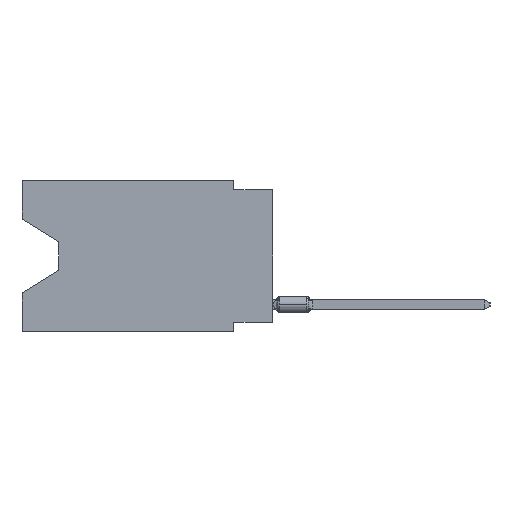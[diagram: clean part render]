
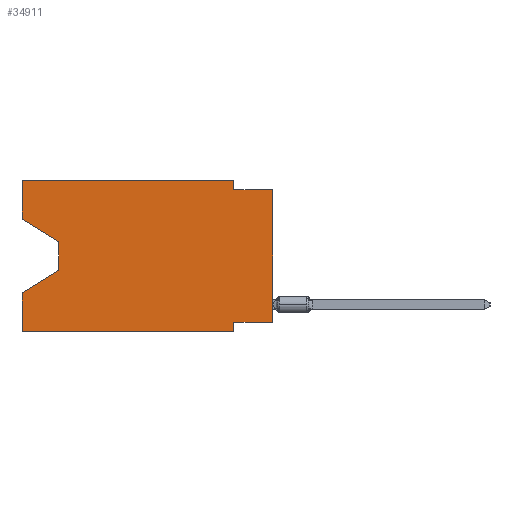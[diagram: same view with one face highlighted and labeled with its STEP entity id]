
A CAD part, left-side view. The second image highlights one B-rep face of the part: STEP entity #34911.
In plain terms, the highlighted planar face has unit normal (-1, 0, 0).
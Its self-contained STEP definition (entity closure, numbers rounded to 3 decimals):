
#473 = LINE ( 'NONE', #30649, #62997 ) ;
#828 = LINE ( 'NONE', #5421, #24261 ) ;
#2259 = CARTESIAN_POINT ( 'NONE',  ( 0., 16.383, -9.906 ) ) ;
#2526 = EDGE_CURVE ( 'NONE', #58920, #43027, #473, .T. ) ;
#2875 = EDGE_LOOP ( 'NONE', ( #43694, #42628, #30547, #45548, #38217, #61983, #20829, #27153, #55555, #23919, #49147, #15992 ) ) ;
#4630 = AXIS2_PLACEMENT_3D ( 'NONE', #52921, #58157, #6998 ) ;
#5217 = CARTESIAN_POINT ( 'NONE',  ( 0., 0., -9.271 ) ) ;
#5275 = CARTESIAN_POINT ( 'NONE',  ( 0., 2.54, -9.271 ) ) ;
#5421 = CARTESIAN_POINT ( 'NONE',  ( 0., 16.383, -9.906 ) ) ;
#6998 = DIRECTION ( 'NONE',  ( 0., 0., -1. ) ) ;
#7374 = CARTESIAN_POINT ( 'NONE',  ( 0., 2.54, -0.635 ) ) ;
#9024 = VECTOR ( 'NONE', #23249, 1000. ) ;
#9771 = LINE ( 'NONE', #28488, #11224 ) ;
#11224 = VECTOR ( 'NONE', #63599, 1000. ) ;
#12387 = VERTEX_POINT ( 'NONE', #34326 ) ;
#12640 = LINE ( 'NONE', #47424, #46484 ) ;
#13572 = CARTESIAN_POINT ( 'NONE',  ( 0., 16.383, 0. ) ) ;
#15992 = ORIENTED_EDGE ( 'NONE', *, *, #59181, .F. ) ;
#16686 = EDGE_CURVE ( 'NONE', #19550, #50573, #31820, .T. ) ;
#17005 = EDGE_CURVE ( 'NONE', #12387, #58920, #42849, .T. ) ;
#18121 = LINE ( 'NONE', #46999, #53094 ) ;
#18966 = EDGE_CURVE ( 'NONE', #30955, #43027, #60913, .T. ) ;
#19330 = EDGE_CURVE ( 'NONE', #64260, #62810, #18121, .T. ) ;
#19540 = CARTESIAN_POINT ( 'NONE',  ( 0., 13.97, -5.893 ) ) ;
#19550 = VERTEX_POINT ( 'NONE', #5275 ) ;
#19842 = VERTEX_POINT ( 'NONE', #48868 ) ;
#20419 = DIRECTION ( 'NONE',  ( 0., 0., 1. ) ) ;
#20829 = ORIENTED_EDGE ( 'NONE', *, *, #53485, .F. ) ;
#23249 = DIRECTION ( 'NONE',  ( 0., 0., -1. ) ) ;
#23919 = ORIENTED_EDGE ( 'NONE', *, *, #59705, .F. ) ;
#24261 = VECTOR ( 'NONE', #46091, 1000. ) ;
#25249 = LINE ( 'NONE', #35106, #38712 ) ;
#26458 = CARTESIAN_POINT ( 'NONE',  ( 0., 16.383, 0. ) ) ;
#27153 = ORIENTED_EDGE ( 'NONE', *, *, #36392, .T. ) ;
#27766 = DIRECTION ( 'NONE',  ( 0., 0., -1. ) ) ;
#28488 = CARTESIAN_POINT ( 'NONE',  ( 0., 16.383, -2.546 ) ) ;
#29995 = VECTOR ( 'NONE', #41547, 1000. ) ;
#30547 = ORIENTED_EDGE ( 'NONE', *, *, #2526, .T. ) ;
#30649 = CARTESIAN_POINT ( 'NONE',  ( 0., 13.97, -5.893 ) ) ;
#30955 = VERTEX_POINT ( 'NONE', #2259 ) ;
#31820 = LINE ( 'NONE', #53140, #9024 ) ;
#32658 = CARTESIAN_POINT ( 'NONE',  ( 0., 0., 0. ) ) ;
#32902 = FACE_OUTER_BOUND ( 'NONE', #2875, .T. ) ;
#33018 = VERTEX_POINT ( 'NONE', #5217 ) ;
#33603 = CARTESIAN_POINT ( 'NONE',  ( 0., 16.383, -2.546 ) ) ;
#34326 = CARTESIAN_POINT ( 'NONE',  ( 0., 13.97, -4.013 ) ) ;
#34911 = ADVANCED_FACE ( 'NONE', ( #32902 ), #51954, .F. ) ;
#35106 = CARTESIAN_POINT ( 'NONE',  ( 0., 2.54, 0. ) ) ;
#36392 = EDGE_CURVE ( 'NONE', #33018, #62810, #63495, .T. ) ;
#36471 = CARTESIAN_POINT ( 'NONE',  ( 0., 2.54, 0. ) ) ;
#38217 = ORIENTED_EDGE ( 'NONE', *, *, #47095, .T. ) ;
#38712 = VECTOR ( 'NONE', #64325, 1000. ) ;
#41398 = CARTESIAN_POINT ( 'NONE',  ( 0., 16.383, -7.36 ) ) ;
#41547 = DIRECTION ( 'NONE',  ( 0., 0., 1. ) ) ;
#42628 = ORIENTED_EDGE ( 'NONE', *, *, #17005, .T. ) ;
#42849 = LINE ( 'NONE', #49643, #60379 ) ;
#43003 = VERTEX_POINT ( 'NONE', #36471 ) ;
#43027 = VERTEX_POINT ( 'NONE', #41398 ) ;
#43694 = ORIENTED_EDGE ( 'NONE', *, *, #56605, .T. ) ;
#44785 = CARTESIAN_POINT ( 'NONE',  ( 0., 0., -0.635 ) ) ;
#44975 = VECTOR ( 'NONE', #20419, 1000. ) ;
#45038 = LINE ( 'NONE', #55525, #44975 ) ;
#45548 = ORIENTED_EDGE ( 'NONE', *, *, #18966, .F. ) ;
#46091 = DIRECTION ( 'NONE',  ( 0., -1., 0. ) ) ;
#46484 = VECTOR ( 'NONE', #61535, 1000. ) ;
#46999 = CARTESIAN_POINT ( 'NONE',  ( 0., 0., -0.635 ) ) ;
#47095 = EDGE_CURVE ( 'NONE', #30955, #50573, #828, .T. ) ;
#47335 = EDGE_CURVE ( 'NONE', #19842, #43003, #49970, .T. ) ;
#47424 = CARTESIAN_POINT ( 'NONE',  ( 0., 0., -9.271 ) ) ;
#48868 = CARTESIAN_POINT ( 'NONE',  ( 0., 16.383, 0. ) ) ;
#49147 = ORIENTED_EDGE ( 'NONE', *, *, #47335, .F. ) ;
#49643 = CARTESIAN_POINT ( 'NONE',  ( 0., 13.97, -4.013 ) ) ;
#49970 = LINE ( 'NONE', #13572, #63085 ) ;
#50573 = VERTEX_POINT ( 'NONE', #62209 ) ;
#51934 = DIRECTION ( 'NONE',  ( 0., -1., 0. ) ) ;
#51954 = PLANE ( 'NONE',  #4630 ) ;
#52921 = CARTESIAN_POINT ( 'NONE',  ( 0., 16.383, 0. ) ) ;
#53094 = VECTOR ( 'NONE', #51934, 1000. ) ;
#53140 = CARTESIAN_POINT ( 'NONE',  ( 0., 2.54, -9.906 ) ) ;
#53485 = EDGE_CURVE ( 'NONE', #33018, #19550, #12640, .T. ) ;
#54248 = DIRECTION ( 'NONE',  ( 0., -1., 0. ) ) ;
#54960 = VECTOR ( 'NONE', #62513, 1000. ) ;
#55525 = CARTESIAN_POINT ( 'NONE',  ( 0., 16.383, 0. ) ) ;
#55555 = ORIENTED_EDGE ( 'NONE', *, *, #19330, .F. ) ;
#56605 = EDGE_CURVE ( 'NONE', #59106, #12387, #9771, .T. ) ;
#58157 = DIRECTION ( 'NONE',  ( 1., 0., 0. ) ) ;
#58920 = VERTEX_POINT ( 'NONE', #19540 ) ;
#59106 = VERTEX_POINT ( 'NONE', #33603 ) ;
#59181 = EDGE_CURVE ( 'NONE', #59106, #19842, #45038, .T. ) ;
#59705 = EDGE_CURVE ( 'NONE', #43003, #64260, #25249, .T. ) ;
#60379 = VECTOR ( 'NONE', #27766, 1000. ) ;
#60495 = DIRECTION ( 'NONE',  ( 0., 0.855, -0.519 ) ) ;
#60913 = LINE ( 'NONE', #26458, #29995 ) ;
#61535 = DIRECTION ( 'NONE',  ( 0., 1., 0. ) ) ;
#61983 = ORIENTED_EDGE ( 'NONE', *, *, #16686, .F. ) ;
#62209 = CARTESIAN_POINT ( 'NONE',  ( 0., 2.54, -9.906 ) ) ;
#62513 = DIRECTION ( 'NONE',  ( 0., 0., 1. ) ) ;
#62810 = VERTEX_POINT ( 'NONE', #44785 ) ;
#62997 = VECTOR ( 'NONE', #60495, 1000. ) ;
#63085 = VECTOR ( 'NONE', #54248, 1000. ) ;
#63495 = LINE ( 'NONE', #32658, #54960 ) ;
#63599 = DIRECTION ( 'NONE',  ( 0., -0.855, -0.519 ) ) ;
#64260 = VERTEX_POINT ( 'NONE', #7374 ) ;
#64325 = DIRECTION ( 'NONE',  ( 0., 0., -1. ) ) ;
